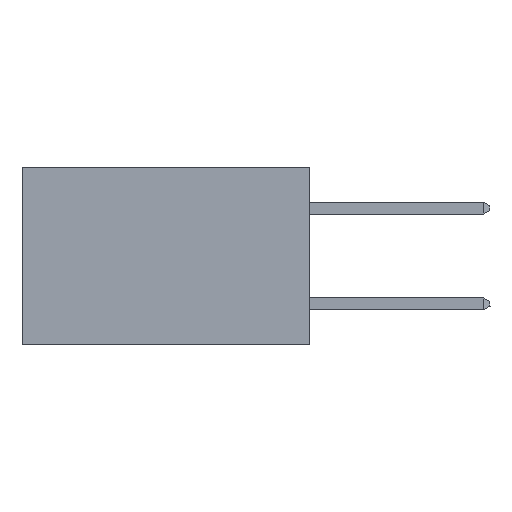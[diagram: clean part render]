
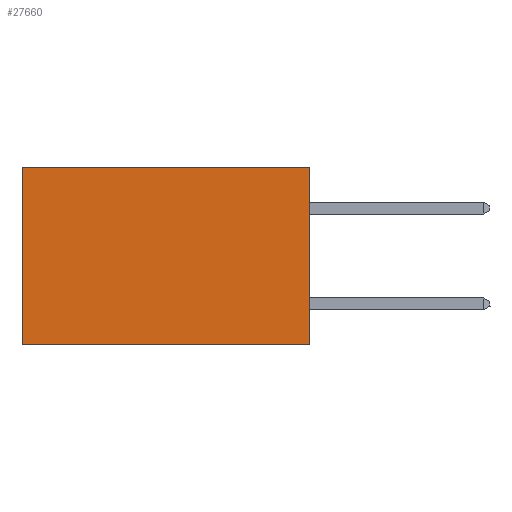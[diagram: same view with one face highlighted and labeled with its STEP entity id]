
A CAD part, left-side view. The second image highlights one B-rep face of the part: STEP entity #27660.
In plain terms, the highlighted planar face has unit normal (-1, 0, 0).
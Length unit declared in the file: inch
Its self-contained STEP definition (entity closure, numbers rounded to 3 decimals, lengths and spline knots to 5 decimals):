
#355 = FACE_OUTER_BOUND ( 'NONE', #5017, .T. ) ;
#1872 = DIRECTION ( 'NONE',  ( 0., 1., 0. ) ) ;
#2328 = ORIENTED_EDGE ( 'NONE', *, *, #4921, .F. ) ;
#3641 = EDGE_CURVE ( 'NONE', #26366, #4365, #11461, .T. ) ;
#4365 = VERTEX_POINT ( 'NONE', #26533 ) ;
#4921 = EDGE_CURVE ( 'NONE', #9880, #14294, #9199, .T. ) ;
#5017 = EDGE_LOOP ( 'NONE', ( #17611, #13533, #2328, #15725 ) ) ;
#5086 = DIRECTION ( 'NONE',  ( 1., 0., 0. ) ) ;
#6156 = CARTESIAN_POINT ( 'NONE',  ( 0.2875, 0., 0. ) ) ;
#6282 = CARTESIAN_POINT ( 'NONE',  ( 0.2875, 0., 0. ) ) ;
#7227 = PLANE ( 'NONE',  #12619 ) ;
#9199 = LINE ( 'NONE', #6282, #14948 ) ;
#9880 = VERTEX_POINT ( 'NONE', #6156 ) ;
#9951 = CARTESIAN_POINT ( 'NONE',  ( 0.2875, 0.6, 0. ) ) ;
#11461 = LINE ( 'NONE', #26579, #16522 ) ;
#12619 = AXIS2_PLACEMENT_3D ( 'NONE', #26605, #5086, #20316 ) ;
#12893 = CARTESIAN_POINT ( 'NONE',  ( 0.2875, 0., 0. ) ) ;
#12934 = CARTESIAN_POINT ( 'NONE',  ( 0.2875, 0., -0.37 ) ) ;
#13324 = LINE ( 'NONE', #12893, #15340 ) ;
#13533 = ORIENTED_EDGE ( 'NONE', *, *, #14170, .F. ) ;
#14170 = EDGE_CURVE ( 'NONE', #14294, #4365, #26897, .T. ) ;
#14294 = VERTEX_POINT ( 'NONE', #21857 ) ;
#14948 = VECTOR ( 'NONE', #27449, 39.37008 ) ;
#15097 = DIRECTION ( 'NONE',  ( 0., 1., 0. ) ) ;
#15340 = VECTOR ( 'NONE', #1872, 39.37008 ) ;
#15725 = ORIENTED_EDGE ( 'NONE', *, *, #16018, .T. ) ;
#16018 = EDGE_CURVE ( 'NONE', #9880, #26366, #13324, .T. ) ;
#16522 = VECTOR ( 'NONE', #20617, 39.37008 ) ;
#17611 = ORIENTED_EDGE ( 'NONE', *, *, #3641, .T. ) ;
#20316 = DIRECTION ( 'NONE',  ( 0., 0., -1. ) ) ;
#20617 = DIRECTION ( 'NONE',  ( 0., 0., -1. ) ) ;
#21857 = CARTESIAN_POINT ( 'NONE',  ( 0.2875, 0., -0.37 ) ) ;
#26202 = VECTOR ( 'NONE', #15097, 39.37008 ) ;
#26366 = VERTEX_POINT ( 'NONE', #9951 ) ;
#26533 = CARTESIAN_POINT ( 'NONE',  ( 0.2875, 0.6, -0.37 ) ) ;
#26579 = CARTESIAN_POINT ( 'NONE',  ( 0.2875, 0.6, 0. ) ) ;
#26605 = CARTESIAN_POINT ( 'NONE',  ( 0.2875, 0., 0. ) ) ;
#26897 = LINE ( 'NONE', #12934, #26202 ) ;
#27449 = DIRECTION ( 'NONE',  ( 0., 0., -1. ) ) ;
#27660 = ADVANCED_FACE ( 'NONE', ( #355 ), #7227, .F. ) ;
